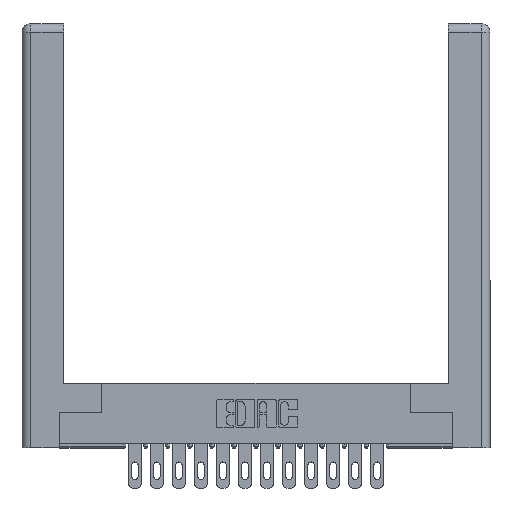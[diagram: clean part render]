
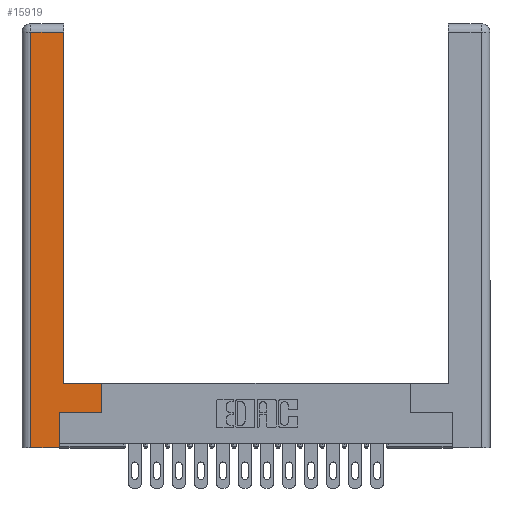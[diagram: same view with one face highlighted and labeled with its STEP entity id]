
A CAD part, top view. The second image highlights one B-rep face of the part: STEP entity #15919.
In plain terms, the highlighted planar face has unit normal (0, 0, 1).
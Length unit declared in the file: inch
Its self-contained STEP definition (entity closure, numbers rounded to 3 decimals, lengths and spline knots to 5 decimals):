
#4 = LINE ( 'NONE', #17523, #17255 ) ;
#848 = CARTESIAN_POINT ( 'NONE',  ( 0.265, 0., 0. ) ) ;
#1224 = VERTEX_POINT ( 'NONE', #9788 ) ;
#1378 = PLANE ( 'NONE',  #7539 ) ;
#1599 = ORIENTED_EDGE ( 'NONE', *, *, #9773, .T. ) ;
#2106 = CARTESIAN_POINT ( 'NONE',  ( 0.295, 3., 0. ) ) ;
#2321 = CARTESIAN_POINT ( 'NONE',  ( 0.565, 0.45, 0. ) ) ;
#2421 = EDGE_CURVE ( 'NONE', #3391, #4601, #4, .T. ) ;
#3075 = VECTOR ( 'NONE', #12018, 39.37008 ) ;
#3391 = VERTEX_POINT ( 'NONE', #16109 ) ;
#4268 = DIRECTION ( 'NONE',  ( 1., 0., 0. ) ) ;
#4568 = DIRECTION ( 'NONE',  ( -1., 0., 0. ) ) ;
#4581 = LINE ( 'NONE', #4920, #12042 ) ;
#4601 = VERTEX_POINT ( 'NONE', #12228 ) ;
#4867 = EDGE_CURVE ( 'NONE', #12984, #1224, #4581, .T. ) ;
#4920 = CARTESIAN_POINT ( 'NONE',  ( 0.295, 0.45, 0. ) ) ;
#4956 = DIRECTION ( 'NONE',  ( 0., 1., 0. ) ) ;
#5292 = CARTESIAN_POINT ( 'NONE',  ( 0.565, 0.245, 0. ) ) ;
#5654 = DIRECTION ( 'NONE',  ( 0., -1., 0. ) ) ;
#5871 = VERTEX_POINT ( 'NONE', #15808 ) ;
#6487 = DIRECTION ( 'NONE',  ( -1., 0., 0. ) ) ;
#6706 = LINE ( 'NONE', #2106, #16501 ) ;
#7042 = LINE ( 'NONE', #9014, #3075 ) ;
#7539 = AXIS2_PLACEMENT_3D ( 'NONE', #13369, #10514, #4568 ) ;
#7574 = LINE ( 'NONE', #2321, #7795 ) ;
#7795 = VECTOR ( 'NONE', #18749, 39.37008 ) ;
#8377 = EDGE_CURVE ( 'NONE', #4601, #19038, #17006, .T. ) ;
#9014 = CARTESIAN_POINT ( 'NONE',  ( 0.0615, 2.94, 0. ) ) ;
#9044 = VERTEX_POINT ( 'NONE', #5292 ) ;
#9502 = DIRECTION ( 'NONE',  ( 0., 1., 0. ) ) ;
#9650 = CARTESIAN_POINT ( 'NONE',  ( 0.295, 2.94, 0. ) ) ;
#9773 = EDGE_CURVE ( 'NONE', #5871, #9044, #10424, .T. ) ;
#9788 = CARTESIAN_POINT ( 'NONE',  ( 0.295, 0.45, 0. ) ) ;
#9881 = VERTEX_POINT ( 'NONE', #9650 ) ;
#10424 = LINE ( 'NONE', #13025, #12314 ) ;
#10514 = DIRECTION ( 'NONE',  ( 0., 0., -1. ) ) ;
#10830 = ORIENTED_EDGE ( 'NONE', *, *, #13667, .T. ) ;
#11636 = EDGE_CURVE ( 'NONE', #9044, #12984, #7574, .T. ) ;
#11736 = VECTOR ( 'NONE', #9502, 39.37008 ) ;
#12018 = DIRECTION ( 'NONE',  ( -1., 0., 0. ) ) ;
#12042 = VECTOR ( 'NONE', #6487, 39.37008 ) ;
#12146 = ORIENTED_EDGE ( 'NONE', *, *, #2421, .T. ) ;
#12228 = CARTESIAN_POINT ( 'NONE',  ( 0.0615, 0., 0. ) ) ;
#12305 = ORIENTED_EDGE ( 'NONE', *, *, #11636, .T. ) ;
#12314 = VECTOR ( 'NONE', #14661, 39.37008 ) ;
#12984 = VERTEX_POINT ( 'NONE', #14406 ) ;
#13025 = CARTESIAN_POINT ( 'NONE',  ( 0.565, 0.245, 0. ) ) ;
#13369 = CARTESIAN_POINT ( 'NONE',  ( 0., 0., 0. ) ) ;
#13667 = EDGE_CURVE ( 'NONE', #19038, #5871, #17550, .T. ) ;
#14030 = CARTESIAN_POINT ( 'NONE',  ( 0.265, 0.245, 0. ) ) ;
#14252 = EDGE_CURVE ( 'NONE', #9881, #3391, #7042, .T. ) ;
#14406 = CARTESIAN_POINT ( 'NONE',  ( 0.565, 0.45, 0. ) ) ;
#14661 = DIRECTION ( 'NONE',  ( 1., 0., 0. ) ) ;
#14839 = ORIENTED_EDGE ( 'NONE', *, *, #14252, .T. ) ;
#15601 = ORIENTED_EDGE ( 'NONE', *, *, #8377, .T. ) ;
#15808 = CARTESIAN_POINT ( 'NONE',  ( 0.265, 0.245, 0. ) ) ;
#15861 = VECTOR ( 'NONE', #4268, 39.37008 ) ;
#15919 = ADVANCED_FACE ( 'NONE', ( #17012 ), #1378, .F. ) ;
#16109 = CARTESIAN_POINT ( 'NONE',  ( 0.0615, 2.94, 0. ) ) ;
#16286 = CARTESIAN_POINT ( 'NONE',  ( 0.265, 0., 0. ) ) ;
#16343 = EDGE_LOOP ( 'NONE', ( #17110, #14839, #12146, #15601, #10830, #1599, #12305, #18738 ) ) ;
#16501 = VECTOR ( 'NONE', #4956, 39.37008 ) ;
#16903 = EDGE_CURVE ( 'NONE', #1224, #9881, #6706, .T. ) ;
#17006 = LINE ( 'NONE', #848, #15861 ) ;
#17012 = FACE_OUTER_BOUND ( 'NONE', #16343, .T. ) ;
#17110 = ORIENTED_EDGE ( 'NONE', *, *, #16903, .T. ) ;
#17255 = VECTOR ( 'NONE', #5654, 39.37008 ) ;
#17523 = CARTESIAN_POINT ( 'NONE',  ( 0.0615, 0., 0. ) ) ;
#17550 = LINE ( 'NONE', #14030, #11736 ) ;
#18738 = ORIENTED_EDGE ( 'NONE', *, *, #4867, .T. ) ;
#18749 = DIRECTION ( 'NONE',  ( 0., 1., 0. ) ) ;
#19038 = VERTEX_POINT ( 'NONE', #16286 ) ;
